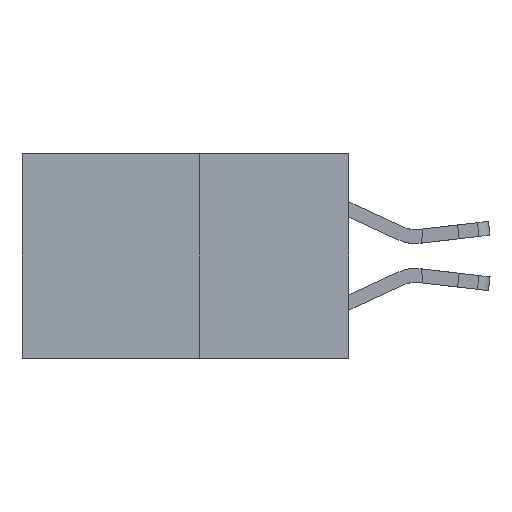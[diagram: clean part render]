
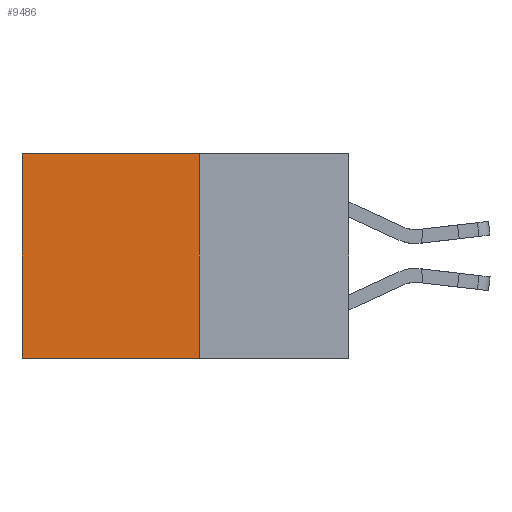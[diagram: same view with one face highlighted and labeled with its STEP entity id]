
A CAD part, left-side view. The second image highlights one B-rep face of the part: STEP entity #9486.
In plain terms, the highlighted planar face has unit normal (-1, 0, 0).
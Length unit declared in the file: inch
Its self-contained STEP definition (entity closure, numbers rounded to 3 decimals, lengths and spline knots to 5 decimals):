
#278 = PLANE ( 'NONE',  #9410 ) ;
#1784 = DIRECTION ( 'NONE',  ( 0., 0., -1. ) ) ;
#1936 = CARTESIAN_POINT ( 'NONE',  ( 0.277, 0.27, -0.37 ) ) ;
#2035 = CARTESIAN_POINT ( 'NONE',  ( 0.277, 0.59, 0. ) ) ;
#3397 = FACE_OUTER_BOUND ( 'NONE', #8351, .T. ) ;
#4285 = LINE ( 'NONE', #16309, #8048 ) ;
#4913 = LINE ( 'NONE', #5292, #8640 ) ;
#5292 = CARTESIAN_POINT ( 'NONE',  ( 0.277, 0.27, -0.37 ) ) ;
#5429 = CARTESIAN_POINT ( 'NONE',  ( 0.277, 0.27, -0.37 ) ) ;
#5895 = DIRECTION ( 'NONE',  ( 0., 1., 0. ) ) ;
#6047 = VECTOR ( 'NONE', #5895, 39.37008 ) ;
#6487 = VERTEX_POINT ( 'NONE', #16189 ) ;
#6899 = DIRECTION ( 'NONE',  ( 0., 0., -1. ) ) ;
#7029 = DIRECTION ( 'NONE',  ( 0., 0., -1. ) ) ;
#8048 = VECTOR ( 'NONE', #8614, 39.37008 ) ;
#8307 = ORIENTED_EDGE ( 'NONE', *, *, #17306, .T. ) ;
#8351 = EDGE_LOOP ( 'NONE', ( #12657, #10981, #19615, #8307 ) ) ;
#8614 = DIRECTION ( 'NONE',  ( 0., 1., 0. ) ) ;
#8640 = VECTOR ( 'NONE', #6899, 39.37008 ) ;
#8784 = LINE ( 'NONE', #14369, #15553 ) ;
#9410 = AXIS2_PLACEMENT_3D ( 'NONE', #5429, #16308, #7029 ) ;
#9486 = ADVANCED_FACE ( 'NONE', ( #3397 ), #278, .F. ) ;
#9738 = LINE ( 'NONE', #16758, #6047 ) ;
#9841 = CARTESIAN_POINT ( 'NONE',  ( 0.277, 0.59, -0.37 ) ) ;
#10981 = ORIENTED_EDGE ( 'NONE', *, *, #12278, .F. ) ;
#12278 = EDGE_CURVE ( 'NONE', #19243, #19884, #9738, .T. ) ;
#12657 = ORIENTED_EDGE ( 'NONE', *, *, #17124, .T. ) ;
#13908 = EDGE_CURVE ( 'NONE', #6487, #19243, #4913, .T. ) ;
#14369 = CARTESIAN_POINT ( 'NONE',  ( 0.277, 0.59, -0.37 ) ) ;
#15553 = VECTOR ( 'NONE', #1784, 39.37008 ) ;
#16189 = CARTESIAN_POINT ( 'NONE',  ( 0.277, 0.27, 0. ) ) ;
#16308 = DIRECTION ( 'NONE',  ( 1., 0., 0. ) ) ;
#16309 = CARTESIAN_POINT ( 'NONE',  ( 0.277, 0.27, 0. ) ) ;
#16758 = CARTESIAN_POINT ( 'NONE',  ( 0.277, 0.27, -0.37 ) ) ;
#17124 = EDGE_CURVE ( 'NONE', #17970, #19884, #8784, .T. ) ;
#17306 = EDGE_CURVE ( 'NONE', #6487, #17970, #4285, .T. ) ;
#17970 = VERTEX_POINT ( 'NONE', #2035 ) ;
#19243 = VERTEX_POINT ( 'NONE', #1936 ) ;
#19615 = ORIENTED_EDGE ( 'NONE', *, *, #13908, .F. ) ;
#19884 = VERTEX_POINT ( 'NONE', #9841 ) ;
